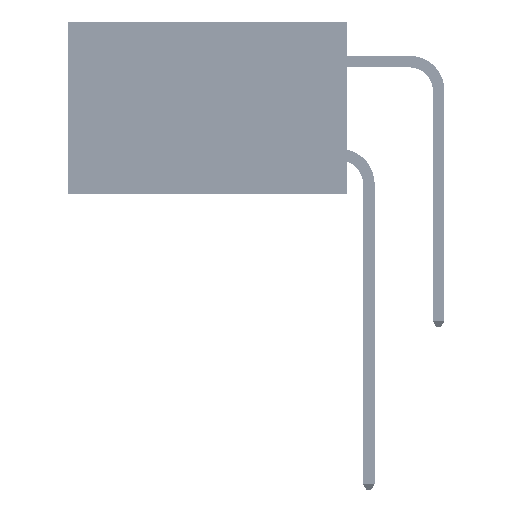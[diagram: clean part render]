
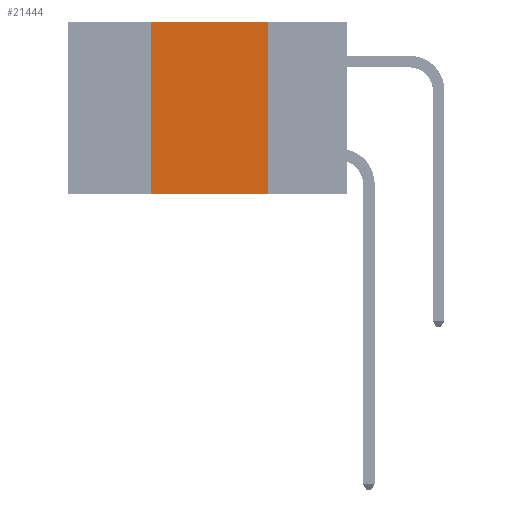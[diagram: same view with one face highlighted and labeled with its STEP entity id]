
A CAD part, left-side view. The second image highlights one B-rep face of the part: STEP entity #21444.
In plain terms, the highlighted planar face has unit normal (-1, 0, 0).
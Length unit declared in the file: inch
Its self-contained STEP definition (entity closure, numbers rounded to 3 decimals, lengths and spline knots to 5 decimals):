
#914 = VECTOR ( 'NONE', #22156, 39.37008 ) ;
#2098 = LINE ( 'NONE', #40429, #914 ) ;
#3708 = CARTESIAN_POINT ( 'NONE',  ( 0., 0.6, 0. ) ) ;
#3769 = FACE_OUTER_BOUND ( 'NONE', #43749, .T. ) ;
#5138 = VERTEX_POINT ( 'NONE', #32056 ) ;
#5237 = CARTESIAN_POINT ( 'NONE',  ( 0., 0.42, 0. ) ) ;
#8585 = VECTOR ( 'NONE', #33293, 39.37008 ) ;
#11860 = LINE ( 'NONE', #21396, #40226 ) ;
#12658 = CARTESIAN_POINT ( 'NONE',  ( 0., 0.6, -0.37 ) ) ;
#12804 = CARTESIAN_POINT ( 'NONE',  ( 0., 0.17, 0. ) ) ;
#15225 = PLANE ( 'NONE',  #35945 ) ;
#15302 = ORIENTED_EDGE ( 'NONE', *, *, #27124, .F. ) ;
#17055 = ORIENTED_EDGE ( 'NONE', *, *, #20427, .T. ) ;
#17332 = VECTOR ( 'NONE', #42270, 39.37008 ) ;
#18881 = ORIENTED_EDGE ( 'NONE', *, *, #21356, .F. ) ;
#19026 = DIRECTION ( 'NONE',  ( 1., 0., 0. ) ) ;
#20427 = EDGE_CURVE ( 'NONE', #41933, #5138, #46743, .T. ) ;
#21356 = EDGE_CURVE ( 'NONE', #25240, #36442, #28579, .T. ) ;
#21396 = CARTESIAN_POINT ( 'NONE',  ( 0., 0.17, 0. ) ) ;
#21444 = ADVANCED_FACE ( 'NONE', ( #3769 ), #15225, .F. ) ;
#22156 = DIRECTION ( 'NONE',  ( 0., 0., 1. ) ) ;
#25240 = VERTEX_POINT ( 'NONE', #5237 ) ;
#27124 = EDGE_CURVE ( 'NONE', #41933, #25240, #2098, .T. ) ;
#28579 = LINE ( 'NONE', #29620, #8585 ) ;
#29497 = EDGE_CURVE ( 'NONE', #36442, #5138, #11860, .T. ) ;
#29620 = CARTESIAN_POINT ( 'NONE',  ( 0., 0.6, 0. ) ) ;
#32056 = CARTESIAN_POINT ( 'NONE',  ( 0., 0.17, -0.37 ) ) ;
#32139 = ORIENTED_EDGE ( 'NONE', *, *, #29497, .F. ) ;
#32430 = DIRECTION ( 'NONE',  ( 0., 0., -1. ) ) ;
#33293 = DIRECTION ( 'NONE',  ( 0., -1., 0. ) ) ;
#33858 = CARTESIAN_POINT ( 'NONE',  ( 0., 0.42, -0.37 ) ) ;
#35945 = AXIS2_PLACEMENT_3D ( 'NONE', #3708, #19026, #44789 ) ;
#36442 = VERTEX_POINT ( 'NONE', #12804 ) ;
#40226 = VECTOR ( 'NONE', #32430, 39.37008 ) ;
#40429 = CARTESIAN_POINT ( 'NONE',  ( 0., 0.42, 0. ) ) ;
#41933 = VERTEX_POINT ( 'NONE', #33858 ) ;
#42270 = DIRECTION ( 'NONE',  ( 0., -1., 0. ) ) ;
#43749 = EDGE_LOOP ( 'NONE', ( #32139, #18881, #15302, #17055 ) ) ;
#44789 = DIRECTION ( 'NONE',  ( 0., 0., -1. ) ) ;
#46743 = LINE ( 'NONE', #12658, #17332 ) ;
